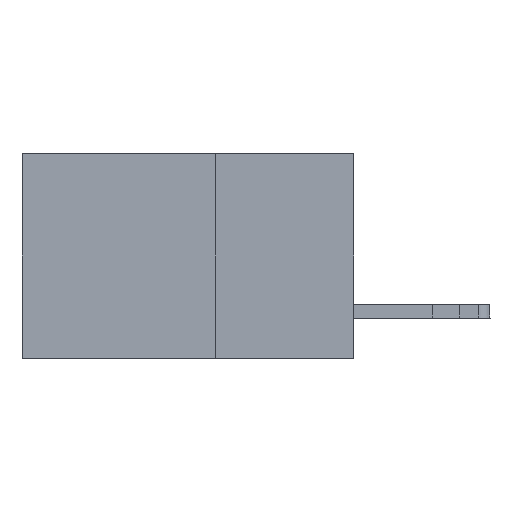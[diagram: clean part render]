
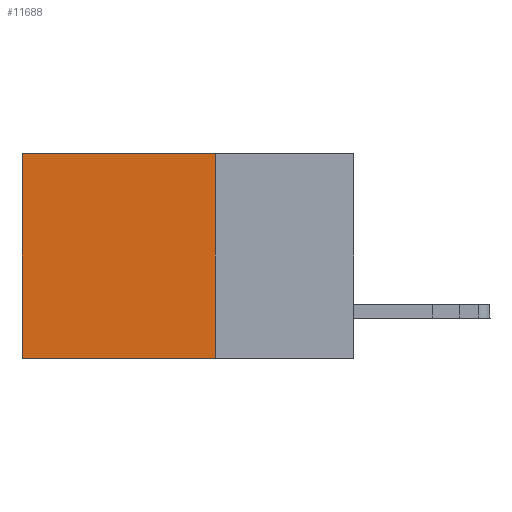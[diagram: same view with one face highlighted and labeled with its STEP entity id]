
A CAD part, left-side view. The second image highlights one B-rep face of the part: STEP entity #11688.
In plain terms, the highlighted planar face has unit normal (-1, 0, 0).
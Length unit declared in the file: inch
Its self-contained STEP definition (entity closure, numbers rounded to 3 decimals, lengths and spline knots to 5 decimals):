
#460 = CARTESIAN_POINT ( 'NONE',  ( 0.2875, 0.25, 0. ) ) ;
#1642 = LINE ( 'NONE', #13142, #18737 ) ;
#2678 = VECTOR ( 'NONE', #23588, 39.37008 ) ;
#3029 = AXIS2_PLACEMENT_3D ( 'NONE', #13196, #16514, #25894 ) ;
#3128 = PLANE ( 'NONE',  #3029 ) ;
#3845 = DIRECTION ( 'NONE',  ( 0., 0., -1. ) ) ;
#5366 = VERTEX_POINT ( 'NONE', #12729 ) ;
#6297 = LINE ( 'NONE', #29821, #25911 ) ;
#6905 = LINE ( 'NONE', #26207, #2678 ) ;
#8401 = CARTESIAN_POINT ( 'NONE',  ( 0.2875, 0.6, 0. ) ) ;
#8553 = EDGE_CURVE ( 'NONE', #29844, #5366, #6905, .T. ) ;
#11688 = ADVANCED_FACE ( 'NONE', ( #29203 ), #3128, .F. ) ;
#12729 = CARTESIAN_POINT ( 'NONE',  ( 0.2875, 0.6, -0.37 ) ) ;
#13142 = CARTESIAN_POINT ( 'NONE',  ( 0.2875, 0.6, 0. ) ) ;
#13196 = CARTESIAN_POINT ( 'NONE',  ( 0.2875, 0.25, 0. ) ) ;
#13715 = ORIENTED_EDGE ( 'NONE', *, *, #20863, .T. ) ;
#13992 = ORIENTED_EDGE ( 'NONE', *, *, #22654, .T. ) ;
#15716 = EDGE_CURVE ( 'NONE', #24780, #29844, #6297, .T. ) ;
#16300 = VECTOR ( 'NONE', #25445, 39.37008 ) ;
#16514 = DIRECTION ( 'NONE',  ( 1., 0., 0. ) ) ;
#18737 = VECTOR ( 'NONE', #18769, 39.37008 ) ;
#18769 = DIRECTION ( 'NONE',  ( 0., 0., -1. ) ) ;
#20380 = EDGE_LOOP ( 'NONE', ( #13992, #25870, #25955, #13715 ) ) ;
#20863 = EDGE_CURVE ( 'NONE', #24780, #21776, #24752, .T. ) ;
#21776 = VERTEX_POINT ( 'NONE', #8401 ) ;
#22654 = EDGE_CURVE ( 'NONE', #21776, #5366, #1642, .T. ) ;
#23588 = DIRECTION ( 'NONE',  ( 0., 1., 0. ) ) ;
#23821 = CARTESIAN_POINT ( 'NONE',  ( 0.2875, 0.25, -0.37 ) ) ;
#24752 = LINE ( 'NONE', #33502, #16300 ) ;
#24780 = VERTEX_POINT ( 'NONE', #460 ) ;
#25445 = DIRECTION ( 'NONE',  ( 0., 1., 0. ) ) ;
#25870 = ORIENTED_EDGE ( 'NONE', *, *, #8553, .F. ) ;
#25894 = DIRECTION ( 'NONE',  ( 0., 0., -1. ) ) ;
#25911 = VECTOR ( 'NONE', #3845, 39.37008 ) ;
#25955 = ORIENTED_EDGE ( 'NONE', *, *, #15716, .F. ) ;
#26207 = CARTESIAN_POINT ( 'NONE',  ( 0.2875, 0.25, -0.37 ) ) ;
#29203 = FACE_OUTER_BOUND ( 'NONE', #20380, .T. ) ;
#29821 = CARTESIAN_POINT ( 'NONE',  ( 0.2875, 0.25, 0. ) ) ;
#29844 = VERTEX_POINT ( 'NONE', #23821 ) ;
#33502 = CARTESIAN_POINT ( 'NONE',  ( 0.2875, 0.25, 0. ) ) ;
